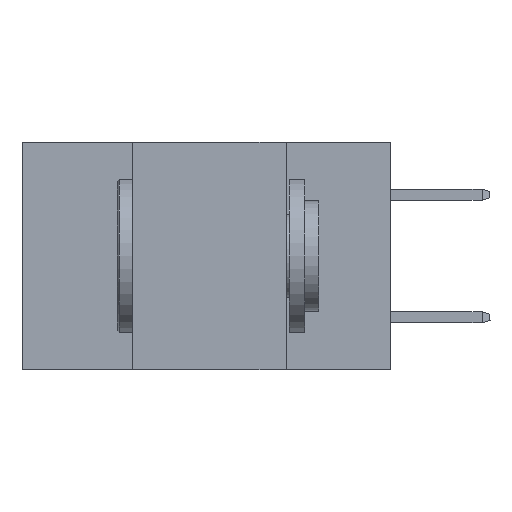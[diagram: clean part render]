
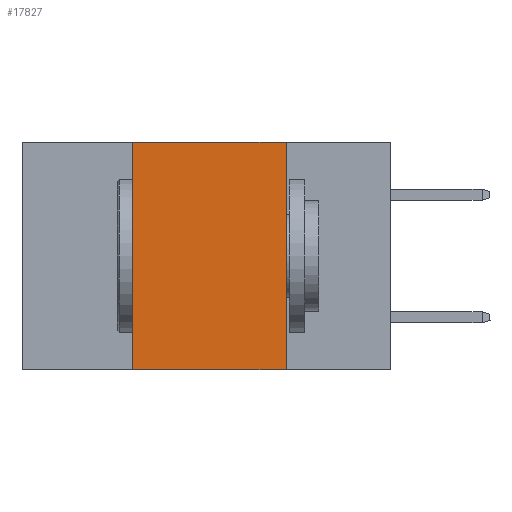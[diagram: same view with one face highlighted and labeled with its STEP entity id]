
A CAD part, left-side view. The second image highlights one B-rep face of the part: STEP entity #17827.
In plain terms, the highlighted planar face has unit normal (-1, 0, 0).
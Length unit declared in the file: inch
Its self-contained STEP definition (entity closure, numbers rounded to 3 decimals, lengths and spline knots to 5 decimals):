
#388 = LINE ( 'NONE', #16191, #17892 ) ;
#1579 = VERTEX_POINT ( 'NONE', #20735 ) ;
#3859 = VERTEX_POINT ( 'NONE', #7649 ) ;
#3927 = DIRECTION ( 'NONE',  ( 0., 0., -1. ) ) ;
#4241 = AXIS2_PLACEMENT_3D ( 'NONE', #9968, #7863, #23655 ) ;
#7371 = DIRECTION ( 'NONE',  ( 0., -1., 0. ) ) ;
#7649 = CARTESIAN_POINT ( 'NONE',  ( 0., 0.17, -0.37 ) ) ;
#7863 = DIRECTION ( 'NONE',  ( 1., 0., 0. ) ) ;
#9488 = LINE ( 'NONE', #19807, #15548 ) ;
#9669 = LINE ( 'NONE', #21979, #26994 ) ;
#9968 = CARTESIAN_POINT ( 'NONE',  ( 0., 0.6, 0. ) ) ;
#10275 = ORIENTED_EDGE ( 'NONE', *, *, #12892, .F. ) ;
#11574 = DIRECTION ( 'NONE',  ( 0., -1., 0. ) ) ;
#12892 = EDGE_CURVE ( 'NONE', #1579, #28548, #9669, .T. ) ;
#13458 = ORIENTED_EDGE ( 'NONE', *, *, #18086, .F. ) ;
#14032 = CARTESIAN_POINT ( 'NONE',  ( 0., 0.6, -0.37 ) ) ;
#14694 = VERTEX_POINT ( 'NONE', #23524 ) ;
#15548 = VECTOR ( 'NONE', #3927, 39.37008 ) ;
#15730 = EDGE_CURVE ( 'NONE', #1579, #3859, #19496, .T. ) ;
#16191 = CARTESIAN_POINT ( 'NONE',  ( 0., 0.6, 0. ) ) ;
#17827 = ADVANCED_FACE ( 'NONE', ( #17995 ), #19159, .F. ) ;
#17892 = VECTOR ( 'NONE', #11574, 39.37008 ) ;
#17995 = FACE_OUTER_BOUND ( 'NONE', #28067, .T. ) ;
#18086 = EDGE_CURVE ( 'NONE', #14694, #3859, #9488, .T. ) ;
#18777 = VECTOR ( 'NONE', #7371, 39.37008 ) ;
#19159 = PLANE ( 'NONE',  #4241 ) ;
#19496 = LINE ( 'NONE', #14032, #18777 ) ;
#19608 = CARTESIAN_POINT ( 'NONE',  ( 0., 0.42, 0. ) ) ;
#19807 = CARTESIAN_POINT ( 'NONE',  ( 0., 0.17, 0. ) ) ;
#20735 = CARTESIAN_POINT ( 'NONE',  ( 0., 0.42, -0.37 ) ) ;
#20994 = ORIENTED_EDGE ( 'NONE', *, *, #25161, .F. ) ;
#21979 = CARTESIAN_POINT ( 'NONE',  ( 0., 0.42, 0. ) ) ;
#23077 = ORIENTED_EDGE ( 'NONE', *, *, #15730, .T. ) ;
#23524 = CARTESIAN_POINT ( 'NONE',  ( 0., 0.17, 0. ) ) ;
#23655 = DIRECTION ( 'NONE',  ( 0., 0., -1. ) ) ;
#25161 = EDGE_CURVE ( 'NONE', #28548, #14694, #388, .T. ) ;
#26842 = DIRECTION ( 'NONE',  ( 0., 0., 1. ) ) ;
#26994 = VECTOR ( 'NONE', #26842, 39.37008 ) ;
#28067 = EDGE_LOOP ( 'NONE', ( #13458, #20994, #10275, #23077 ) ) ;
#28548 = VERTEX_POINT ( 'NONE', #19608 ) ;
